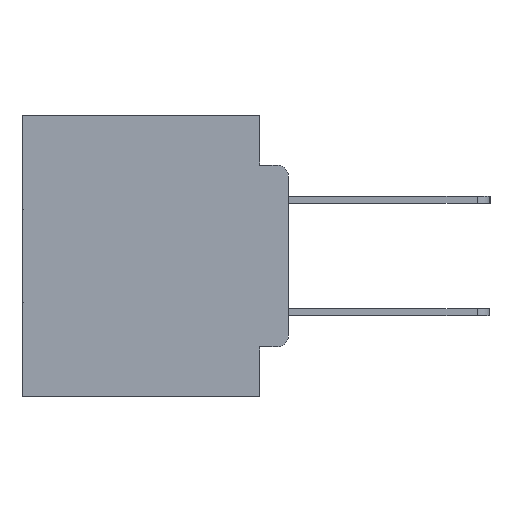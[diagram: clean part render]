
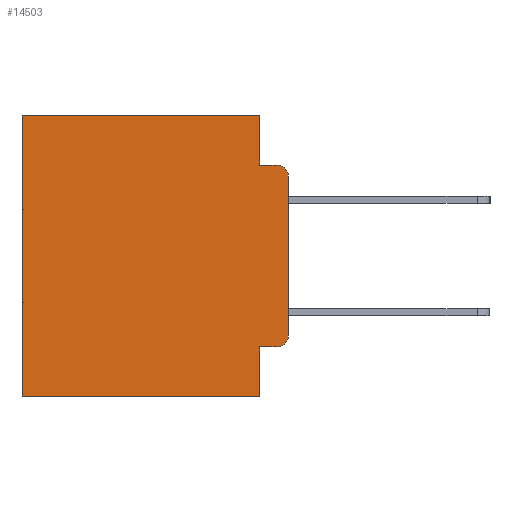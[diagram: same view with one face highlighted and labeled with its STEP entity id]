
A CAD part, left-side view. The second image highlights one B-rep face of the part: STEP entity #14503.
In plain terms, the highlighted planar face has unit normal (-1, 0, 0).
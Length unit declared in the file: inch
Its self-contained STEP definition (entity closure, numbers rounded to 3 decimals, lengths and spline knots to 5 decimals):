
#324 = VECTOR ( 'NONE', #11022, 39.37008 ) ;
#679 = ORIENTED_EDGE ( 'NONE', *, *, #825, .T. ) ;
#698 = VECTOR ( 'NONE', #2263, 39.37008 ) ;
#825 = EDGE_CURVE ( 'NONE', #12575, #30815, #7651, .T. ) ;
#1013 = LINE ( 'NONE', #12443, #14166 ) ;
#1029 = EDGE_CURVE ( 'NONE', #2876, #4212, #8819, .T. ) ;
#2186 = CARTESIAN_POINT ( 'NONE',  ( 0.298, 0., 0. ) ) ;
#2263 = DIRECTION ( 'NONE',  ( 0., 0., -1. ) ) ;
#2433 = VECTOR ( 'NONE', #30416, 39.37008 ) ;
#2701 = EDGE_CURVE ( 'NONE', #25737, #2876, #28779, .T. ) ;
#2876 = VERTEX_POINT ( 'NONE', #3800 ) ;
#3800 = CARTESIAN_POINT ( 'NONE',  ( 0.298, 0.02, -0.4115 ) ) ;
#4212 = VERTEX_POINT ( 'NONE', #12481 ) ;
#4342 = EDGE_CURVE ( 'NONE', #25737, #27557, #27547, .T. ) ;
#4655 = DIRECTION ( 'NONE',  ( 1., 0., 0. ) ) ;
#4932 = AXIS2_PLACEMENT_3D ( 'NONE', #26247, #11694, #28676 ) ;
#5011 = ORIENTED_EDGE ( 'NONE', *, *, #2701, .T. ) ;
#6053 = EDGE_CURVE ( 'NONE', #30815, #27375, #1013, .T. ) ;
#6502 = ORIENTED_EDGE ( 'NONE', *, *, #11027, .T. ) ;
#7523 = AXIS2_PLACEMENT_3D ( 'NONE', #2186, #4655, #21850 ) ;
#7651 = LINE ( 'NONE', #11524, #19144 ) ;
#7709 = EDGE_CURVE ( 'NONE', #12575, #31041, #9055, .T. ) ;
#7738 = ORIENTED_EDGE ( 'NONE', *, *, #4342, .F. ) ;
#7777 = LINE ( 'NONE', #28007, #324 ) ;
#8629 = ORIENTED_EDGE ( 'NONE', *, *, #14285, .F. ) ;
#8646 = VERTEX_POINT ( 'NONE', #19602 ) ;
#8819 = CIRCLE ( 'NONE', #31048, 0.02 ) ;
#8910 = VECTOR ( 'NONE', #13662, 39.37008 ) ;
#9055 = LINE ( 'NONE', #11469, #2433 ) ;
#9375 = EDGE_CURVE ( 'NONE', #31041, #8646, #12229, .T. ) ;
#9407 = VECTOR ( 'NONE', #12741, 39.37008 ) ;
#11022 = DIRECTION ( 'NONE',  ( 0., 1., 0. ) ) ;
#11027 = EDGE_CURVE ( 'NONE', #12632, #8646, #19022, .T. ) ;
#11204 = ORIENTED_EDGE ( 'NONE', *, *, #13693, .F. ) ;
#11469 = CARTESIAN_POINT ( 'NONE',  ( 0.298, 0.051, 0. ) ) ;
#11524 = CARTESIAN_POINT ( 'NONE',  ( 0.298, 0., 0. ) ) ;
#11694 = DIRECTION ( 'NONE',  ( -1., 0., 0. ) ) ;
#12229 = LINE ( 'NONE', #19530, #25937 ) ;
#12348 = CARTESIAN_POINT ( 'NONE',  ( 0.298, 0.051, -0.5 ) ) ;
#12443 = CARTESIAN_POINT ( 'NONE',  ( 0.298, 0.473, 0. ) ) ;
#12481 = CARTESIAN_POINT ( 'NONE',  ( 0.298, 0., -0.3915 ) ) ;
#12575 = VERTEX_POINT ( 'NONE', #27657 ) ;
#12632 = VERTEX_POINT ( 'NONE', #25449 ) ;
#12645 = CARTESIAN_POINT ( 'NONE',  ( 0.298, 0.051, -0.4115 ) ) ;
#12741 = DIRECTION ( 'NONE',  ( 0., -1., 0. ) ) ;
#13662 = DIRECTION ( 'NONE',  ( 0., 0., -1. ) ) ;
#13693 = EDGE_CURVE ( 'NONE', #27557, #27375, #7777, .T. ) ;
#14166 = VECTOR ( 'NONE', #15323, 39.37008 ) ;
#14285 = EDGE_CURVE ( 'NONE', #12632, #4212, #16227, .T. ) ;
#14503 = ADVANCED_FACE ( 'NONE', ( #29415 ), #28995, .F. ) ;
#14586 = CARTESIAN_POINT ( 'NONE',  ( 0.298, 0.051, -0.4115 ) ) ;
#14973 = CARTESIAN_POINT ( 'NONE',  ( 0.298, 0.473, 0. ) ) ;
#15323 = DIRECTION ( 'NONE',  ( 0., 0., -1. ) ) ;
#15422 = ORIENTED_EDGE ( 'NONE', *, *, #6053, .T. ) ;
#15937 = CARTESIAN_POINT ( 'NONE',  ( 0.298, 0.051, -0.0885 ) ) ;
#16227 = LINE ( 'NONE', #25866, #8910 ) ;
#16568 = DIRECTION ( 'NONE',  ( 0., 0., -1. ) ) ;
#17678 = DIRECTION ( 'NONE',  ( -1., 0., 0. ) ) ;
#18349 = CARTESIAN_POINT ( 'NONE',  ( 0.298, 0.473, -0.5 ) ) ;
#19022 = CIRCLE ( 'NONE', #4932, 0.02 ) ;
#19144 = VECTOR ( 'NONE', #31078, 39.37008 ) ;
#19309 = CARTESIAN_POINT ( 'NONE',  ( 0.298, 0.02, -0.3915 ) ) ;
#19530 = CARTESIAN_POINT ( 'NONE',  ( 0.298, 0.051, -0.0885 ) ) ;
#19602 = CARTESIAN_POINT ( 'NONE',  ( 0.298, 0.02, -0.0885 ) ) ;
#19621 = ORIENTED_EDGE ( 'NONE', *, *, #9375, .F. ) ;
#21548 = DIRECTION ( 'NONE',  ( 0., -1., 0. ) ) ;
#21850 = DIRECTION ( 'NONE',  ( 0., 0., -1. ) ) ;
#22830 = EDGE_LOOP ( 'NONE', ( #8629, #6502, #19621, #23393, #679, #15422, #11204, #7738, #5011, #26774 ) ) ;
#23393 = ORIENTED_EDGE ( 'NONE', *, *, #7709, .F. ) ;
#25449 = CARTESIAN_POINT ( 'NONE',  ( 0.298, 0., -0.1085 ) ) ;
#25737 = VERTEX_POINT ( 'NONE', #14586 ) ;
#25866 = CARTESIAN_POINT ( 'NONE',  ( 0.298, 0., 0. ) ) ;
#25937 = VECTOR ( 'NONE', #21548, 39.37008 ) ;
#26247 = CARTESIAN_POINT ( 'NONE',  ( 0.298, 0.02, -0.1085 ) ) ;
#26774 = ORIENTED_EDGE ( 'NONE', *, *, #1029, .T. ) ;
#27375 = VERTEX_POINT ( 'NONE', #18349 ) ;
#27547 = LINE ( 'NONE', #30258, #698 ) ;
#27557 = VERTEX_POINT ( 'NONE', #12348 ) ;
#27657 = CARTESIAN_POINT ( 'NONE',  ( 0.298, 0.051, 0. ) ) ;
#28007 = CARTESIAN_POINT ( 'NONE',  ( 0.298, 0., -0.5 ) ) ;
#28676 = DIRECTION ( 'NONE',  ( 0., 0., -1. ) ) ;
#28779 = LINE ( 'NONE', #12645, #9407 ) ;
#28995 = PLANE ( 'NONE',  #7523 ) ;
#29415 = FACE_OUTER_BOUND ( 'NONE', #22830, .T. ) ;
#30258 = CARTESIAN_POINT ( 'NONE',  ( 0.298, 0.051, 0. ) ) ;
#30416 = DIRECTION ( 'NONE',  ( 0., 0., -1. ) ) ;
#30815 = VERTEX_POINT ( 'NONE', #14973 ) ;
#31041 = VERTEX_POINT ( 'NONE', #15937 ) ;
#31048 = AXIS2_PLACEMENT_3D ( 'NONE', #19309, #17678, #16568 ) ;
#31078 = DIRECTION ( 'NONE',  ( 0., 1., 0. ) ) ;
